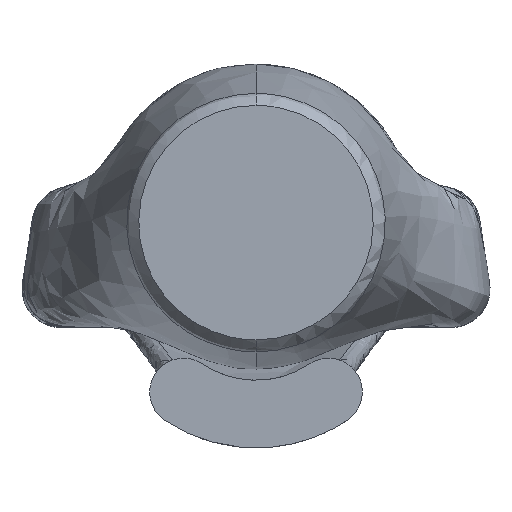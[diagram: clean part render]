
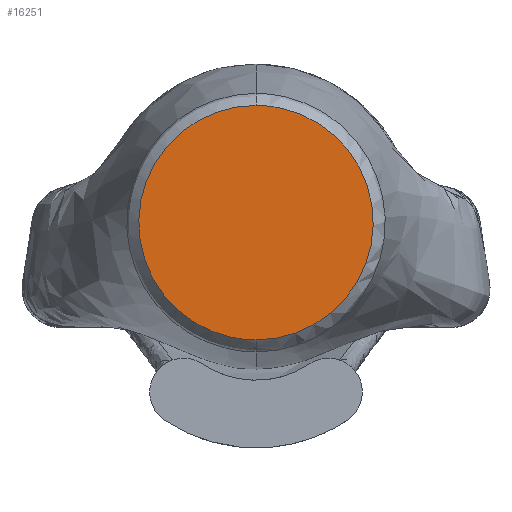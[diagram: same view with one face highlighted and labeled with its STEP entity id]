
A CAD part, top view. The second image highlights one B-rep face of the part: STEP entity #16251.
In plain terms, the highlighted planar face has unit normal (0, 0, 1).
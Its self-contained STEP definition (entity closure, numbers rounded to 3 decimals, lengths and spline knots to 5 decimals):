
#58 = CARTESIAN_POINT ( 'NONE',  ( 0.05234, -0.17253, 0.8 ) ) ;
#71 = CARTESIAN_POINT ( 'NONE',  ( -0.13936, 0.11437, 0.8 ) ) ;
#2732 = DIRECTION ( 'NONE',  ( 0., 0., 1. ) ) ;
#3269 = CARTESIAN_POINT ( 'NONE',  ( -0.069, 0.16657, 0.8 ) ) ;
#3782 = CARTESIAN_POINT ( 'NONE',  ( -0.16658, -0.069, 0.8 ) ) ;
#4034 = CARTESIAN_POINT ( 'NONE',  ( 0., -0.18, 0.8 ) ) ;
#4047 = CARTESIAN_POINT ( 'NONE',  ( -0.03517, -0.17683, 0.8 ) ) ;
#4296 = CARTESIAN_POINT ( 'NONE',  ( 0.17942, 0.01767, 0.8 ) ) ;
#4556 = CARTESIAN_POINT ( 'NONE',  ( 0.00589, 0.18, 0.8 ) ) ;
#4812 = CARTESIAN_POINT ( 'NONE',  ( 0.08499, 0.159, 0.8 ) ) ;
#7244 = CARTESIAN_POINT ( 'NONE',  ( -0.1499, -0.10016, 0.8 ) ) ;
#7758 = CARTESIAN_POINT ( 'NONE',  ( -0.17253, -0.05234, 0.8 ) ) ;
#7969 = ORIENTED_EDGE ( 'NONE', *, *, #18819, .T. ) ;
#8021 = CARTESIAN_POINT ( 'NONE',  ( 0., 0.18, 0.8 ) ) ;
#8273 = CARTESIAN_POINT ( 'NONE',  ( 0.10016, -0.1499, 0.8 ) ) ;
#8286 = CARTESIAN_POINT ( 'NONE',  ( -0.11438, 0.13937, 0.8 ) ) ;
#8539 = CARTESIAN_POINT ( 'NONE',  ( 0.01767, -0.17942, 0.8 ) ) ;
#11213 = CARTESIAN_POINT ( 'NONE',  ( -0.02945, 0.17827, 0.8 ) ) ;
#11720 = CARTESIAN_POINT ( 'NONE',  ( 0.11438, -0.13937, 0.8 ) ) ;
#11732 = CARTESIAN_POINT ( 'NONE',  ( -0.12749, -0.12749, 0.8 ) ) ;
#11979 = CARTESIAN_POINT ( 'NONE',  ( 0.17253, -0.05234, 0.8 ) ) ;
#12253 = CARTESIAN_POINT ( 'NONE',  ( -0.159, 0.08499, 0.8 ) ) ;
#12766 = CARTESIAN_POINT ( 'NONE',  ( 0.12749, 0.12749, 0.8 ) ) ;
#13272 = CARTESIAN_POINT ( 'NONE',  ( 0., 0.18, 0.8 ) ) ;
#13533 = CARTESIAN_POINT ( 'NONE',  ( 0.159, 0.08499, 0.8 ) ) ;
#13791 = CARTESIAN_POINT ( 'NONE',  ( 0.069, 0.16657, 0.8 ) ) ;
#15449 = CARTESIAN_POINT ( 'NONE',  ( -0.08499, 0.159, 0.8 ) ) ;
#15707 = CARTESIAN_POINT ( 'NONE',  ( -0.10016, -0.1499, 0.8 ) ) ;
#15974 = CARTESIAN_POINT ( 'NONE',  ( -0.12749, 0.12749, 0.8 ) ) ;
#16219 = CARTESIAN_POINT ( 'NONE',  ( 0.08499, -0.159, 0.8 ) ) ;
#16251 = ADVANCED_FACE ( 'NONE', ( #26835 ), #42755, .T. ) ;
#16742 = CARTESIAN_POINT ( 'NONE',  ( 0.16658, 0.069, 0.8 ) ) ;
#18191 = ORIENTED_EDGE ( 'NONE', *, *, #46051, .T. ) ;
#18819 = EDGE_CURVE ( 'NONE', #44492, #31814, #44113, .T. ) ;
#18891 = DIRECTION ( 'NONE',  ( 1., 0., 0. ) ) ;
#19427 = CARTESIAN_POINT ( 'NONE',  ( -0.1499, 0.10016, 0.8 ) ) ;
#19713 = B_SPLINE_CURVE_WITH_KNOTS ( 'NONE', 3,
 ( #4034, #35838, #8539, #48049, #58, #51773, #16219, #8273, #11720, #36627, #27875, #44066, #32120, #48309, #11979, #28396, #28134, #24425, #4296, #28922, #33670, #16742, #13533, #33408, #45367, #12766, #45627, #32898, #4812, #13791, #41644, #50118, #29176, #4556, #13272 ),
 .UNSPECIFIED., .F., .F.,
 ( 4, 1, 1, 1, 1, 1, 1, 1, 1, 1, 1, 1, 1, 1, 1, 1, 1, 1, 1, 1, 1, 1, 1, 1, 1, 1, 1, 1, 1, 1, 1, 1, 4 ),
 ( 0.01449, 0.01495, 0.0154, 0.01585, 0.0163, 0.01676, 0.01721, 0.01766, 0.01812, 0.01857, 0.01902, 0.01947, 0.01993, 0.02038, 0.02083, 0.02128, 0.02174, 0.02219, 0.02264, 0.0231, 0.02355, 0.024, 0.02445, 0.02491, 0.02536, 0.02581, 0.02626, 0.02672, 0.02717, 0.02762, 0.02808, 0.02853, 0.02898 ),
 .UNSPECIFIED. ) ;
#19945 = CARTESIAN_POINT ( 'NONE',  ( -0.159, -0.08499, 0.8 ) ) ;
#23394 = CARTESIAN_POINT ( 'NONE',  ( -0.05234, -0.17253, 0.8 ) ) ;
#23652 = CARTESIAN_POINT ( 'NONE',  ( -0.01178, 0.18, 0.8 ) ) ;
#24172 = CARTESIAN_POINT ( 'NONE',  ( -0.17942, -0.01767, 0.8 ) ) ;
#24425 = CARTESIAN_POINT ( 'NONE',  ( 0.1803, 0., 0.8 ) ) ;
#24438 = CARTESIAN_POINT ( 'NONE',  ( -0.16658, 0.069, 0.8 ) ) ;
#26835 = FACE_OUTER_BOUND ( 'NONE', #27586, .T. ) ;
#27372 = CARTESIAN_POINT ( 'NONE',  ( -0.05234, 0.17253, 0.8 ) ) ;
#27586 = EDGE_LOOP ( 'NONE', ( #7969, #18191 ) ) ;
#27875 = CARTESIAN_POINT ( 'NONE',  ( 0.13936, -0.11437, 0.8 ) ) ;
#27888 = CARTESIAN_POINT ( 'NONE',  ( -0.069, -0.16657, 0.8 ) ) ;
#28134 = CARTESIAN_POINT ( 'NONE',  ( 0.17942, -0.01767, 0.8 ) ) ;
#28147 = CARTESIAN_POINT ( 'NONE',  ( -0.10016, 0.1499, 0.8 ) ) ;
#28396 = CARTESIAN_POINT ( 'NONE',  ( 0.17682, -0.03517, 0.8 ) ) ;
#28409 = CARTESIAN_POINT ( 'NONE',  ( -0.17682, -0.03517, 0.8 ) ) ;
#28922 = CARTESIAN_POINT ( 'NONE',  ( 0.17682, 0.03517, 0.8 ) ) ;
#29176 = CARTESIAN_POINT ( 'NONE',  ( 0.01767, 0.17942, 0.8 ) ) ;
#31607 = CARTESIAN_POINT ( 'NONE',  ( -0.00589, -0.18, 0.8 ) ) ;
#31814 = VERTEX_POINT ( 'NONE', #33515 ) ;
#31866 = CARTESIAN_POINT ( 'NONE',  ( -0.17942, 0.01767, 0.8 ) ) ;
#32120 = CARTESIAN_POINT ( 'NONE',  ( 0.159, -0.08499, 0.8 ) ) ;
#32133 = CARTESIAN_POINT ( 'NONE',  ( -0.11438, -0.13937, 0.8 ) ) ;
#32392 = CARTESIAN_POINT ( 'NONE',  ( -0.01767, -0.17942, 0.8 ) ) ;
#32898 = CARTESIAN_POINT ( 'NONE',  ( 0.10016, 0.1499, 0.8 ) ) ;
#33408 = CARTESIAN_POINT ( 'NONE',  ( 0.1499, 0.10016, 0.8 ) ) ;
#33515 = CARTESIAN_POINT ( 'NONE',  ( 0., -0.18, 0.8 ) ) ;
#33670 = CARTESIAN_POINT ( 'NONE',  ( 0.17253, 0.05234, 0.8 ) ) ;
#35591 = CARTESIAN_POINT ( 'NONE',  ( -0.17682, 0.03517, 0.8 ) ) ;
#35838 = CARTESIAN_POINT ( 'NONE',  ( 0.00589, -0.18, 0.8 ) ) ;
#36627 = CARTESIAN_POINT ( 'NONE',  ( 0.12749, -0.12749, 0.8 ) ) ;
#40396 = AXIS2_PLACEMENT_3D ( 'NONE', #46477, #2732, #18891 ) ;
#41644 = CARTESIAN_POINT ( 'NONE',  ( 0.05234, 0.17253, 0.8 ) ) ;
#42755 = PLANE ( 'NONE',  #40396 ) ;
#43151 = CARTESIAN_POINT ( 'NONE',  ( 0., 0.18, 0.8 ) ) ;
#43563 = CARTESIAN_POINT ( 'NONE',  ( -0.17253, 0.05234, 0.8 ) ) ;
#44066 = CARTESIAN_POINT ( 'NONE',  ( 0.1499, -0.10016, 0.8 ) ) ;
#44078 = CARTESIAN_POINT ( 'NONE',  ( -0.1803, 0., 0.8 ) ) ;
#44113 = B_SPLINE_CURVE_WITH_KNOTS ( 'NONE', 3,
 ( #8021, #23652, #11213, #27372, #3269, #15449, #28147, #8286, #15974, #71, #19427, #12253, #24438, #43563, #35591, #31866, #44078, #24172, #28409, #7758, #3782, #19945, #7244, #48060, #11732, #32133, #15707, #44342, #27888, #23394, #4047, #32392, #31607, #47804 ),
 .UNSPECIFIED., .F., .F.,
 ( 4, 1, 1, 1, 1, 1, 1, 1, 1, 1, 1, 1, 1, 1, 1, 1, 1, 1, 1, 1, 1, 1, 1, 1, 1, 1, 1, 1, 1, 1, 1, 4 ),
 ( 0., 0.00091, 0.00136, 0.00181, 0.00226, 0.00272, 0.00317, 0.00362, 0.00408, 0.00453, 0.00498, 0.00544, 0.00589, 0.00634, 0.00679, 0.00725, 0.0077, 0.00815, 0.00861, 0.00906, 0.00951, 0.00996, 0.01042, 0.01087, 0.01132, 0.01178, 0.01223, 0.01268, 0.01314, 0.01359, 0.01404, 0.01449 ),
 .UNSPECIFIED. ) ;
#44342 = CARTESIAN_POINT ( 'NONE',  ( -0.08499, -0.159, 0.8 ) ) ;
#44492 = VERTEX_POINT ( 'NONE', #43151 ) ;
#45367 = CARTESIAN_POINT ( 'NONE',  ( 0.13936, 0.11437, 0.8 ) ) ;
#45627 = CARTESIAN_POINT ( 'NONE',  ( 0.11438, 0.13937, 0.8 ) ) ;
#46051 = EDGE_CURVE ( 'NONE', #31814, #44492, #19713, .T. ) ;
#46477 = CARTESIAN_POINT ( 'NONE',  ( 0., 0., 0.8 ) ) ;
#47804 = CARTESIAN_POINT ( 'NONE',  ( 0., -0.18, 0.8 ) ) ;
#48049 = CARTESIAN_POINT ( 'NONE',  ( 0.03517, -0.17683, 0.8 ) ) ;
#48060 = CARTESIAN_POINT ( 'NONE',  ( -0.13936, -0.11437, 0.8 ) ) ;
#48309 = CARTESIAN_POINT ( 'NONE',  ( 0.16658, -0.069, 0.8 ) ) ;
#50118 = CARTESIAN_POINT ( 'NONE',  ( 0.03517, 0.17683, 0.8 ) ) ;
#51773 = CARTESIAN_POINT ( 'NONE',  ( 0.069, -0.16657, 0.8 ) ) ;
